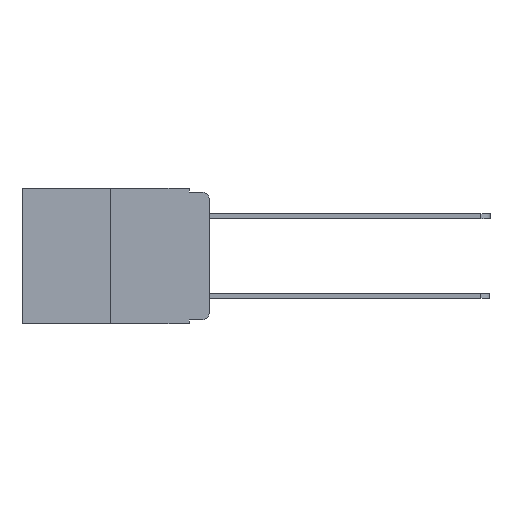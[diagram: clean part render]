
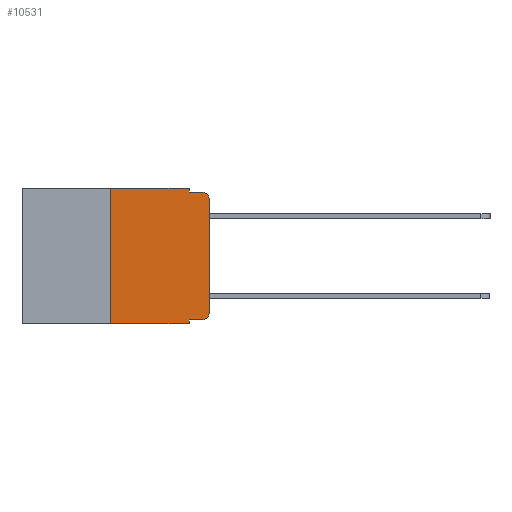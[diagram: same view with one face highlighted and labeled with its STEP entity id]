
A CAD part, left-side view. The second image highlights one B-rep face of the part: STEP entity #10531.
In plain terms, the highlighted planar face has unit normal (-1, 0, 0).
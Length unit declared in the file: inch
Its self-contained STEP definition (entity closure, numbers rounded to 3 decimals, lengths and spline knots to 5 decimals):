
#25 = AXIS2_PLACEMENT_3D ( 'NONE', #4677, #13031, #4738 ) ;
#920 = CIRCLE ( 'NONE', #10340, 0.02 ) ;
#1035 = VERTEX_POINT ( 'NONE', #2468 ) ;
#1359 = EDGE_CURVE ( 'NONE', #1035, #17260, #13917, .T. ) ;
#1392 = VERTEX_POINT ( 'NONE', #7566 ) ;
#1513 = CARTESIAN_POINT ( 'NONE',  ( 0., 0., -0.03 ) ) ;
#1625 = ORIENTED_EDGE ( 'NONE', *, *, #13707, .F. ) ;
#1870 = LINE ( 'NONE', #7211, #12439 ) ;
#2468 = CARTESIAN_POINT ( 'NONE',  ( 0., 0.25, -0.343 ) ) ;
#2597 = LINE ( 'NONE', #9518, #5819 ) ;
#2651 = CARTESIAN_POINT ( 'NONE',  ( 0., 0., 0. ) ) ;
#3014 = DIRECTION ( 'NONE',  ( -1., 0., 0. ) ) ;
#3091 = ORIENTED_EDGE ( 'NONE', *, *, #6651, .T. ) ;
#3123 = EDGE_CURVE ( 'NONE', #17260, #17319, #14401, .T. ) ;
#3199 = CARTESIAN_POINT ( 'NONE',  ( 0., 0., -0.313 ) ) ;
#3345 = VECTOR ( 'NONE', #7380, 39.37008 ) ;
#3841 = LINE ( 'NONE', #12570, #6684 ) ;
#3983 = ORIENTED_EDGE ( 'NONE', *, *, #5916, .T. ) ;
#4022 = DIRECTION ( 'NONE',  ( 0., 0., 1. ) ) ;
#4072 = VERTEX_POINT ( 'NONE', #4345 ) ;
#4192 = ORIENTED_EDGE ( 'NONE', *, *, #12785, .T. ) ;
#4224 = VECTOR ( 'NONE', #13979, 39.37008 ) ;
#4283 = DIRECTION ( 'NONE',  ( 0., 0., -1. ) ) ;
#4345 = CARTESIAN_POINT ( 'NONE',  ( 0., 0.02, -0.333 ) ) ;
#4390 = CARTESIAN_POINT ( 'NONE',  ( 0., 0.051, 0. ) ) ;
#4677 = CARTESIAN_POINT ( 'NONE',  ( 0., 0.473, 0. ) ) ;
#4738 = DIRECTION ( 'NONE',  ( 0., 0., -1. ) ) ;
#5779 = DIRECTION ( 'NONE',  ( 0., 0., -1. ) ) ;
#5819 = VECTOR ( 'NONE', #13694, 39.37008 ) ;
#5916 = EDGE_CURVE ( 'NONE', #4072, #9115, #8475, .T. ) ;
#6651 = EDGE_CURVE ( 'NONE', #7115, #6896, #920, .T. ) ;
#6684 = VECTOR ( 'NONE', #4283, 39.37008 ) ;
#6730 = VERTEX_POINT ( 'NONE', #15916 ) ;
#6896 = VERTEX_POINT ( 'NONE', #7908 ) ;
#6988 = EDGE_CURVE ( 'NONE', #16012, #4072, #2597, .T. ) ;
#7022 = LINE ( 'NONE', #4390, #13931 ) ;
#7115 = VERTEX_POINT ( 'NONE', #1513 ) ;
#7211 = CARTESIAN_POINT ( 'NONE',  ( 0., 0.051, -0.01 ) ) ;
#7380 = DIRECTION ( 'NONE',  ( 0., -1., 0. ) ) ;
#7484 = CARTESIAN_POINT ( 'NONE',  ( 0., 0.02, -0.03 ) ) ;
#7566 = CARTESIAN_POINT ( 'NONE',  ( 0., 0.051, -0.343 ) ) ;
#7837 = CARTESIAN_POINT ( 'NONE',  ( 0., 0.25, 0. ) ) ;
#7908 = CARTESIAN_POINT ( 'NONE',  ( 0., 0.02, -0.01 ) ) ;
#7928 = DIRECTION ( 'NONE',  ( 0., 0., 1. ) ) ;
#7929 = LINE ( 'NONE', #11192, #4224 ) ;
#8009 = CARTESIAN_POINT ( 'NONE',  ( 0., 0.473, 0. ) ) ;
#8475 = CIRCLE ( 'NONE', #15073, 0.02 ) ;
#8734 = ORIENTED_EDGE ( 'NONE', *, *, #16213, .T. ) ;
#8888 = DIRECTION ( 'NONE',  ( 0., 0., -1. ) ) ;
#9115 = VERTEX_POINT ( 'NONE', #3199 ) ;
#9327 = VECTOR ( 'NONE', #4022, 39.37008 ) ;
#9518 = CARTESIAN_POINT ( 'NONE',  ( 0., 0.051, -0.333 ) ) ;
#9748 = LINE ( 'NONE', #2651, #9327 ) ;
#9843 = EDGE_LOOP ( 'NONE', ( #8734, #3091, #10881, #1625, #13070, #10668, #4192, #12862, #13307, #3983 ) ) ;
#10340 = AXIS2_PLACEMENT_3D ( 'NONE', #7484, #17097, #8888 ) ;
#10531 = ADVANCED_FACE ( 'NONE', ( #15770 ), #11626, .F. ) ;
#10629 = CARTESIAN_POINT ( 'NONE',  ( 0., 0.051, 0. ) ) ;
#10668 = ORIENTED_EDGE ( 'NONE', *, *, #1359, .F. ) ;
#10881 = ORIENTED_EDGE ( 'NONE', *, *, #13130, .F. ) ;
#11192 = CARTESIAN_POINT ( 'NONE',  ( 0., 0.473, -0.343 ) ) ;
#11306 = CARTESIAN_POINT ( 'NONE',  ( 0., 0.02, -0.313 ) ) ;
#11503 = EDGE_CURVE ( 'NONE', #16012, #1392, #3841, .T. ) ;
#11626 = PLANE ( 'NONE',  #25 ) ;
#12439 = VECTOR ( 'NONE', #15458, 39.37008 ) ;
#12570 = CARTESIAN_POINT ( 'NONE',  ( 0., 0.051, 0. ) ) ;
#12705 = DIRECTION ( 'NONE',  ( 0., 0., -1. ) ) ;
#12785 = EDGE_CURVE ( 'NONE', #1035, #1392, #7929, .T. ) ;
#12862 = ORIENTED_EDGE ( 'NONE', *, *, #11503, .F. ) ;
#13031 = DIRECTION ( 'NONE',  ( 1., 0., 0. ) ) ;
#13070 = ORIENTED_EDGE ( 'NONE', *, *, #3123, .F. ) ;
#13130 = EDGE_CURVE ( 'NONE', #6730, #6896, #1870, .T. ) ;
#13307 = ORIENTED_EDGE ( 'NONE', *, *, #6988, .T. ) ;
#13694 = DIRECTION ( 'NONE',  ( 0., -1., 0. ) ) ;
#13707 = EDGE_CURVE ( 'NONE', #17319, #6730, #7022, .T. ) ;
#13917 = LINE ( 'NONE', #16724, #16673 ) ;
#13931 = VECTOR ( 'NONE', #5779, 39.37008 ) ;
#13979 = DIRECTION ( 'NONE',  ( 0., -1., 0. ) ) ;
#14401 = LINE ( 'NONE', #8009, #3345 ) ;
#14625 = CARTESIAN_POINT ( 'NONE',  ( 0., 0.051, -0.333 ) ) ;
#15073 = AXIS2_PLACEMENT_3D ( 'NONE', #11306, #3014, #12705 ) ;
#15458 = DIRECTION ( 'NONE',  ( 0., -1., 0. ) ) ;
#15770 = FACE_OUTER_BOUND ( 'NONE', #9843, .T. ) ;
#15916 = CARTESIAN_POINT ( 'NONE',  ( 0., 0.051, -0.01 ) ) ;
#16012 = VERTEX_POINT ( 'NONE', #14625 ) ;
#16213 = EDGE_CURVE ( 'NONE', #9115, #7115, #9748, .T. ) ;
#16673 = VECTOR ( 'NONE', #7928, 39.37008 ) ;
#16724 = CARTESIAN_POINT ( 'NONE',  ( 0., 0.25, 0. ) ) ;
#17097 = DIRECTION ( 'NONE',  ( -1., 0., 0. ) ) ;
#17260 = VERTEX_POINT ( 'NONE', #7837 ) ;
#17319 = VERTEX_POINT ( 'NONE', #10629 ) ;
